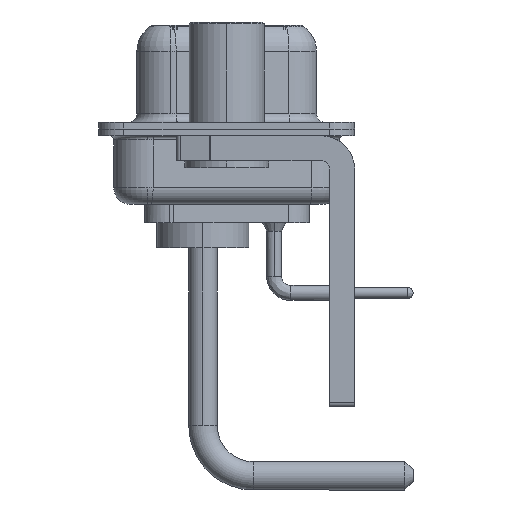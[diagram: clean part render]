
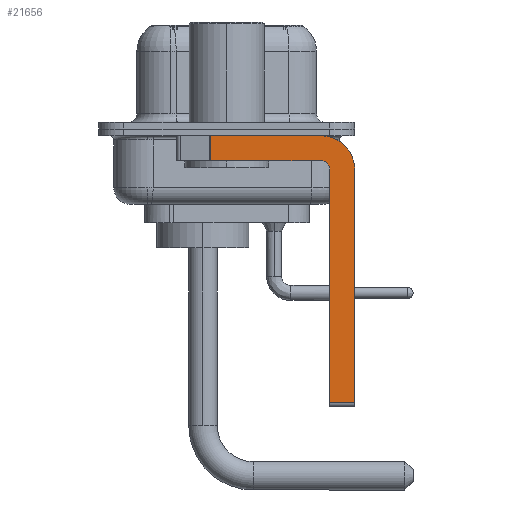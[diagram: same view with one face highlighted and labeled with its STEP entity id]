
A CAD part, left-side view. The second image highlights one B-rep face of the part: STEP entity #21656.
In plain terms, the highlighted planar face has unit normal (-1, 0, 0).
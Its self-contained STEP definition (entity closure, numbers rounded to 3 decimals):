
#167 = DIRECTION ( 'NONE',  ( 0., 0., -1. ) ) ;
#316 = VERTEX_POINT ( 'NONE', #4236 ) ;
#384 = DIRECTION ( 'NONE',  ( 0., 0., -1. ) ) ;
#403 = CARTESIAN_POINT ( 'NONE',  ( -2.9, -5.65, -16.35 ) ) ;
#510 = AXIS2_PLACEMENT_3D ( 'NONE', #8600, #23264, #16274 ) ;
#979 = DIRECTION ( 'NONE',  ( 0., 0., 1. ) ) ;
#1441 = LINE ( 'NONE', #12361, #15768 ) ;
#1754 = EDGE_LOOP ( 'NONE', ( #23130, #3810, #12147, #12733, #2348, #6956, #4837, #19272 ) ) ;
#1841 = EDGE_CURVE ( 'NONE', #15195, #6283, #9527, .T. ) ;
#2348 = ORIENTED_EDGE ( 'NONE', *, *, #3805, .F. ) ;
#2771 = CARTESIAN_POINT ( 'NONE',  ( -2.9, -6.15, -16.6 ) ) ;
#3470 = DIRECTION ( 'NONE',  ( 0., 1., 0. ) ) ;
#3513 = DIRECTION ( 'NONE',  ( 1., 0., 0. ) ) ;
#3805 = EDGE_CURVE ( 'NONE', #23424, #22328, #19215, .T. ) ;
#3810 = ORIENTED_EDGE ( 'NONE', *, *, #15417, .T. ) ;
#3948 = LINE ( 'NONE', #22706, #19114 ) ;
#3991 = VECTOR ( 'NONE', #167, 1000. ) ;
#4236 = CARTESIAN_POINT ( 'NONE',  ( -2.9, 0.978, -1.9 ) ) ;
#4837 = ORIENTED_EDGE ( 'NONE', *, *, #1841, .F. ) ;
#5436 = EDGE_CURVE ( 'NONE', #13921, #15195, #18095, .T. ) ;
#5477 = CIRCLE ( 'NONE', #510, 0.5 ) ;
#6239 = DIRECTION ( 'NONE',  ( 0., -1., 0. ) ) ;
#6283 = VERTEX_POINT ( 'NONE', #19883 ) ;
#6900 = VERTEX_POINT ( 'NONE', #7379 ) ;
#6956 = ORIENTED_EDGE ( 'NONE', *, *, #20408, .T. ) ;
#7225 = EDGE_CURVE ( 'NONE', #6900, #316, #1441, .T. ) ;
#7295 = DIRECTION ( 'NONE',  ( 0., 0., -1. ) ) ;
#7379 = CARTESIAN_POINT ( 'NONE',  ( -2.9, -5.65, -1.9 ) ) ;
#8600 = CARTESIAN_POINT ( 'NONE',  ( -2.9, -5.65, -2.4 ) ) ;
#9505 = DIRECTION ( 'NONE',  ( 1., 0., 0. ) ) ;
#9527 = LINE ( 'NONE', #11085, #3991 ) ;
#9899 = VERTEX_POINT ( 'NONE', #10027 ) ;
#10027 = CARTESIAN_POINT ( 'NONE',  ( -2.9, 0.978, -0.4 ) ) ;
#10215 = VECTOR ( 'NONE', #7295, 1000. ) ;
#10923 = EDGE_CURVE ( 'NONE', #22328, #6900, #5477, .T. ) ;
#11085 = CARTESIAN_POINT ( 'NONE',  ( -2.9, -7.65, -2.4 ) ) ;
#11363 = VECTOR ( 'NONE', #16370, 1000. ) ;
#12147 = ORIENTED_EDGE ( 'NONE', *, *, #7225, .F. ) ;
#12361 = CARTESIAN_POINT ( 'NONE',  ( -2.9, -5.65, -1.9 ) ) ;
#12733 = ORIENTED_EDGE ( 'NONE', *, *, #10923, .F. ) ;
#12973 = CARTESIAN_POINT ( 'NONE',  ( -2.9, -5.65, -2.4 ) ) ;
#13921 = VERTEX_POINT ( 'NONE', #19674 ) ;
#14559 = PLANE ( 'NONE',  #16401 ) ;
#14799 = CARTESIAN_POINT ( 'NONE',  ( -2.9, -6.15, -16.35 ) ) ;
#15195 = VERTEX_POINT ( 'NONE', #19572 ) ;
#15417 = EDGE_CURVE ( 'NONE', #9899, #316, #17964, .T. ) ;
#15478 = CARTESIAN_POINT ( 'NONE',  ( -2.9, -6.15, -2.4 ) ) ;
#15768 = VECTOR ( 'NONE', #3470, 1000. ) ;
#16274 = DIRECTION ( 'NONE',  ( 0., 0., 1. ) ) ;
#16297 = CARTESIAN_POINT ( 'NONE',  ( -2.9, 0.978, -1.9 ) ) ;
#16370 = DIRECTION ( 'NONE',  ( 0., -1., 0. ) ) ;
#16401 = AXIS2_PLACEMENT_3D ( 'NONE', #21894, #3513, #17696 ) ;
#16452 = EDGE_CURVE ( 'NONE', #9899, #13921, #3948, .T. ) ;
#17696 = DIRECTION ( 'NONE',  ( 0., 0., -1. ) ) ;
#17964 = LINE ( 'NONE', #16297, #10215 ) ;
#18095 = CIRCLE ( 'NONE', #21640, 2. ) ;
#18632 = LINE ( 'NONE', #403, #11363 ) ;
#19114 = VECTOR ( 'NONE', #6239, 1000. ) ;
#19215 = LINE ( 'NONE', #2771, #20794 ) ;
#19272 = ORIENTED_EDGE ( 'NONE', *, *, #5436, .F. ) ;
#19572 = CARTESIAN_POINT ( 'NONE',  ( -2.9, -7.65, -2.4 ) ) ;
#19674 = CARTESIAN_POINT ( 'NONE',  ( -2.9, -5.65, -0.4 ) ) ;
#19883 = CARTESIAN_POINT ( 'NONE',  ( -2.9, -7.65, -16.35 ) ) ;
#20408 = EDGE_CURVE ( 'NONE', #23424, #6283, #18632, .T. ) ;
#20794 = VECTOR ( 'NONE', #979, 1000. ) ;
#21640 = AXIS2_PLACEMENT_3D ( 'NONE', #12973, #9505, #384 ) ;
#21656 = ADVANCED_FACE ( 'NONE', ( #23348 ), #14559, .F. ) ;
#21894 = CARTESIAN_POINT ( 'NONE',  ( -2.9, -5.65, -2.4 ) ) ;
#22328 = VERTEX_POINT ( 'NONE', #15478 ) ;
#22706 = CARTESIAN_POINT ( 'NONE',  ( -2.9, 3., -0.4 ) ) ;
#23130 = ORIENTED_EDGE ( 'NONE', *, *, #16452, .F. ) ;
#23264 = DIRECTION ( 'NONE',  ( -1., 0., 0. ) ) ;
#23348 = FACE_OUTER_BOUND ( 'NONE', #1754, .T. ) ;
#23424 = VERTEX_POINT ( 'NONE', #14799 ) ;
